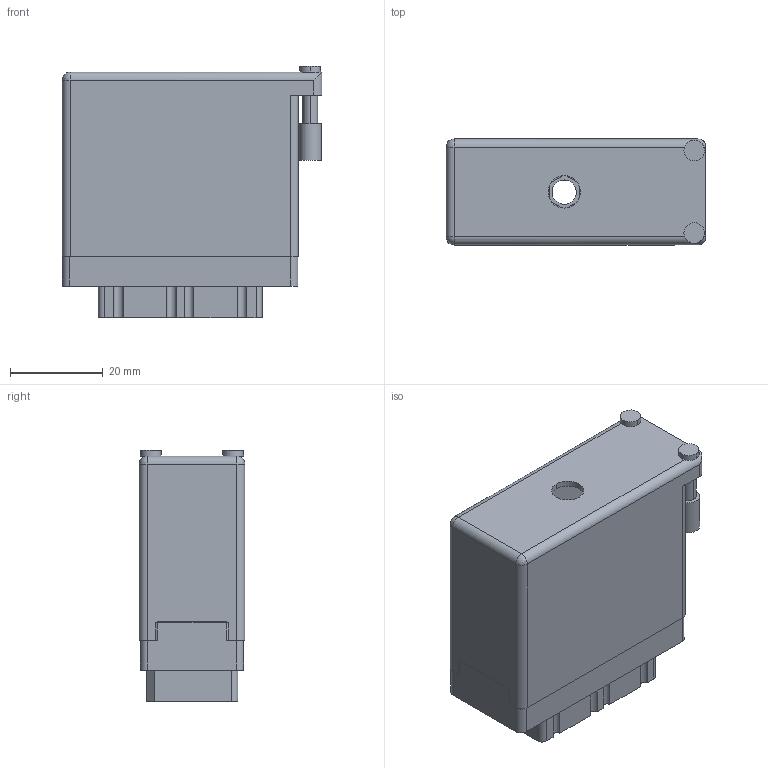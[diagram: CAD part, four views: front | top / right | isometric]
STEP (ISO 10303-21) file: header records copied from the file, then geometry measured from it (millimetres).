
FILE_DESCRIPTION (( 'STEP AP203' ), '1' );
FILE_NAME ('519-036-500-450.STEP', '2020-09-09T20:31:23', ( '' ), ( '' ), 'SwSTEP 2.0', 'SolidWorks 2020', '' );
FILE_SCHEMA (( 'CONFIG_CONTROL_DESIGN' ));
Length unit declared in the file: inch
Products named in the file (4): 519 Receptacle Insulator_036; 516-292-001_500 Contact; 519-036-500-450; 516-230-001_Metal - 038 Side Entry
Assembly tree (38 placements, depth 2):
  519-036-500-450
    519 Receptacle Insulator_036
    516-292-001_500 Contact  x36
    516-230-001_Metal - 038 Side Entry
Bounding box: 56.08 x 22.83 x 54.28 mm (x, y, z)
Volume: 21218.3 mm3; surface area: 34103.9 mm2
Topology: 38 solids, 38 shells, 3645 faces, 10570 edges, 7016 vertices
Faces by surface type: plane 2192, cylinder 1233, bspline 216, cone 2, sphere 2
Entity records: 34481 total; most frequent: CARTESIAN_POINT 6126, ORIENTED_EDGE 5736, DIRECTION 5578, EDGE_CURVE 2868, LINE 2120, VECTOR 2120, VERTEX_POINT 1906, AXIS2_PLACEMENT_3D 1729
